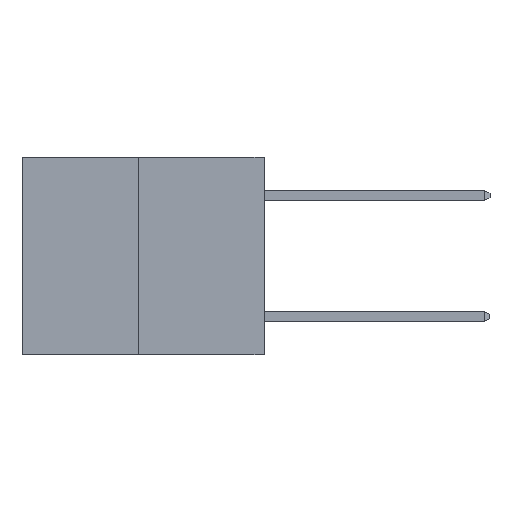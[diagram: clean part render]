
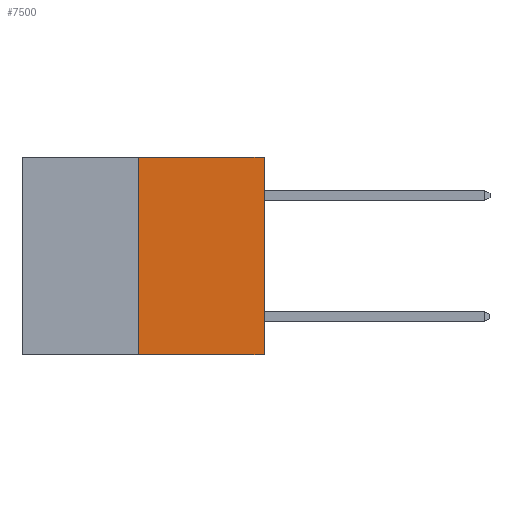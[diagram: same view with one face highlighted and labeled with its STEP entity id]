
A CAD part, left-side view. The second image highlights one B-rep face of the part: STEP entity #7500.
In plain terms, the highlighted planar face has unit normal (-1, 0, 0).
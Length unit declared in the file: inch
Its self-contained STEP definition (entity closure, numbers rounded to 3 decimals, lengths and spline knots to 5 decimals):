
#958 = EDGE_CURVE ( 'NONE', #8728, #13222, #8041, .T. ) ;
#2156 = DIRECTION ( 'NONE',  ( 0., 0., 1. ) ) ;
#2217 = AXIS2_PLACEMENT_3D ( 'NONE', #3221, #13776, #4736 ) ;
#2661 = DIRECTION ( 'NONE',  ( 0., 0., 1. ) ) ;
#2853 = EDGE_CURVE ( 'NONE', #8728, #14056, #9861, .T. ) ;
#3183 = EDGE_CURVE ( 'NONE', #14056, #11238, #13964, .T. ) ;
#3221 = CARTESIAN_POINT ( 'NONE',  ( 0., 0.6, 0. ) ) ;
#4604 = CARTESIAN_POINT ( 'NONE',  ( 0., 0.312, -0.49 ) ) ;
#4736 = DIRECTION ( 'NONE',  ( 0., 0., -1. ) ) ;
#5290 = CARTESIAN_POINT ( 'NONE',  ( 0., 0.6, -0.49 ) ) ;
#5317 = CARTESIAN_POINT ( 'NONE',  ( 0., 0., -0.49 ) ) ;
#5760 = VECTOR ( 'NONE', #18697, 39.37008 ) ;
#6246 = ORIENTED_EDGE ( 'NONE', *, *, #3183, .F. ) ;
#6373 = ORIENTED_EDGE ( 'NONE', *, *, #2853, .F. ) ;
#6791 = LINE ( 'NONE', #11192, #11518 ) ;
#7500 = ADVANCED_FACE ( 'NONE', ( #15242 ), #10751, .F. ) ;
#7594 = ORIENTED_EDGE ( 'NONE', *, *, #958, .T. ) ;
#8041 = LINE ( 'NONE', #5290, #10622 ) ;
#8728 = VERTEX_POINT ( 'NONE', #4604 ) ;
#9518 = EDGE_CURVE ( 'NONE', #13222, #11238, #6791, .T. ) ;
#9861 = LINE ( 'NONE', #11686, #17611 ) ;
#10566 = CARTESIAN_POINT ( 'NONE',  ( 0., 0.312, 0. ) ) ;
#10622 = VECTOR ( 'NONE', #12703, 39.37008 ) ;
#10751 = PLANE ( 'NONE',  #2217 ) ;
#11192 = CARTESIAN_POINT ( 'NONE',  ( 0., 0., 0. ) ) ;
#11238 = VERTEX_POINT ( 'NONE', #17486 ) ;
#11518 = VECTOR ( 'NONE', #2156, 39.37008 ) ;
#11536 = EDGE_LOOP ( 'NONE', ( #6373, #7594, #13422, #6246 ) ) ;
#11686 = CARTESIAN_POINT ( 'NONE',  ( 0., 0.312, -0.49 ) ) ;
#12703 = DIRECTION ( 'NONE',  ( 0., -1., 0. ) ) ;
#13222 = VERTEX_POINT ( 'NONE', #5317 ) ;
#13422 = ORIENTED_EDGE ( 'NONE', *, *, #9518, .T. ) ;
#13776 = DIRECTION ( 'NONE',  ( 1., 0., 0. ) ) ;
#13964 = LINE ( 'NONE', #14232, #5760 ) ;
#14056 = VERTEX_POINT ( 'NONE', #10566 ) ;
#14232 = CARTESIAN_POINT ( 'NONE',  ( 0., 0.6, 0. ) ) ;
#15242 = FACE_OUTER_BOUND ( 'NONE', #11536, .T. ) ;
#17486 = CARTESIAN_POINT ( 'NONE',  ( 0., 0., 0. ) ) ;
#17611 = VECTOR ( 'NONE', #2661, 39.37008 ) ;
#18697 = DIRECTION ( 'NONE',  ( 0., -1., 0. ) ) ;
